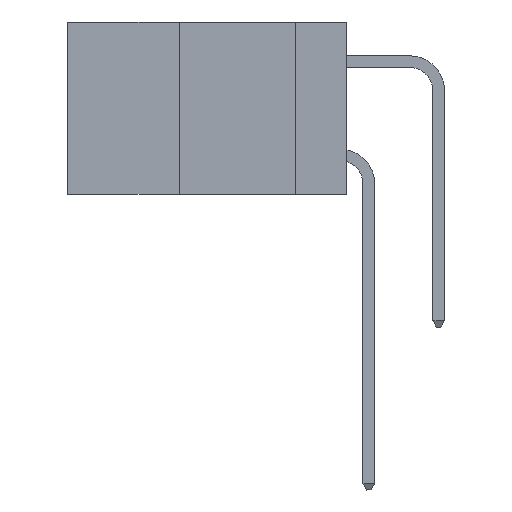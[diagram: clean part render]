
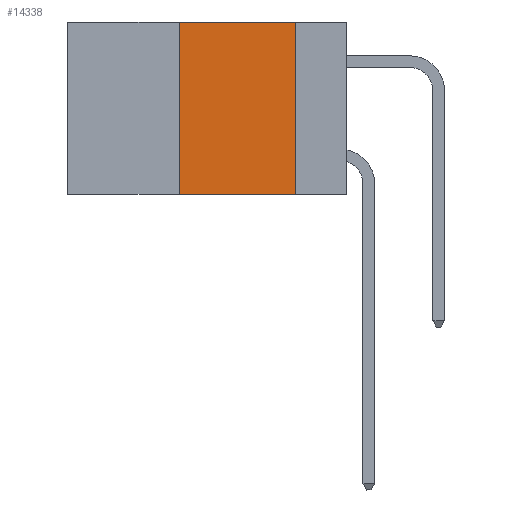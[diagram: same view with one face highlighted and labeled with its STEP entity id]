
A CAD part, left-side view. The second image highlights one B-rep face of the part: STEP entity #14338.
In plain terms, the highlighted planar face has unit normal (-1, 0, 0).
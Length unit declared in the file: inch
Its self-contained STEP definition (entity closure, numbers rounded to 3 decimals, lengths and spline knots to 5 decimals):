
#374 = CARTESIAN_POINT ( 'NONE',  ( 0., 0.36, -0.37 ) ) ;
#404 = VERTEX_POINT ( 'NONE', #2750 ) ;
#1026 = LINE ( 'NONE', #2837, #20509 ) ;
#1184 = ORIENTED_EDGE ( 'NONE', *, *, #21869, .T. ) ;
#1238 = FACE_OUTER_BOUND ( 'NONE', #15495, .T. ) ;
#2445 = LINE ( 'NONE', #23393, #23615 ) ;
#2750 = CARTESIAN_POINT ( 'NONE',  ( 0., 0.11, 0. ) ) ;
#2837 = CARTESIAN_POINT ( 'NONE',  ( 0., 0.11, 0. ) ) ;
#6249 = CARTESIAN_POINT ( 'NONE',  ( 0., 0.6, -0.37 ) ) ;
#6513 = EDGE_CURVE ( 'NONE', #9274, #24567, #2445, .T. ) ;
#6569 = ORIENTED_EDGE ( 'NONE', *, *, #11504, .F. ) ;
#6601 = VERTEX_POINT ( 'NONE', #9102 ) ;
#7382 = DIRECTION ( 'NONE',  ( 0., -1., 0. ) ) ;
#7770 = PLANE ( 'NONE',  #24382 ) ;
#9102 = CARTESIAN_POINT ( 'NONE',  ( 0., 0.11, -0.37 ) ) ;
#9274 = VERTEX_POINT ( 'NONE', #374 ) ;
#9464 = LINE ( 'NONE', #9606, #15316 ) ;
#9606 = CARTESIAN_POINT ( 'NONE',  ( 0., 0.6, 0. ) ) ;
#9864 = DIRECTION ( 'NONE',  ( 1., 0., 0. ) ) ;
#11504 = EDGE_CURVE ( 'NONE', #404, #6601, #1026, .T. ) ;
#13127 = CARTESIAN_POINT ( 'NONE',  ( 0., 0.36, 0. ) ) ;
#14338 = ADVANCED_FACE ( 'NONE', ( #1238 ), #7770, .F. ) ;
#15316 = VECTOR ( 'NONE', #7382, 39.37008 ) ;
#15495 = EDGE_LOOP ( 'NONE', ( #6569, #25408, #18931, #1184 ) ) ;
#18931 = ORIENTED_EDGE ( 'NONE', *, *, #6513, .F. ) ;
#20509 = VECTOR ( 'NONE', #21851, 39.37008 ) ;
#21664 = EDGE_CURVE ( 'NONE', #24567, #404, #9464, .T. ) ;
#21851 = DIRECTION ( 'NONE',  ( 0., 0., -1. ) ) ;
#21869 = EDGE_CURVE ( 'NONE', #9274, #6601, #27304, .T. ) ;
#23393 = CARTESIAN_POINT ( 'NONE',  ( 0., 0.36, 0. ) ) ;
#23615 = VECTOR ( 'NONE', #27380, 39.37008 ) ;
#24382 = AXIS2_PLACEMENT_3D ( 'NONE', #24828, #9864, #24966 ) ;
#24567 = VERTEX_POINT ( 'NONE', #13127 ) ;
#24828 = CARTESIAN_POINT ( 'NONE',  ( 0., 0.6, 0. ) ) ;
#24966 = DIRECTION ( 'NONE',  ( 0., 0., -1. ) ) ;
#25058 = VECTOR ( 'NONE', #25248, 39.37008 ) ;
#25248 = DIRECTION ( 'NONE',  ( 0., -1., 0. ) ) ;
#25408 = ORIENTED_EDGE ( 'NONE', *, *, #21664, .F. ) ;
#27304 = LINE ( 'NONE', #6249, #25058 ) ;
#27380 = DIRECTION ( 'NONE',  ( 0., 0., 1. ) ) ;
